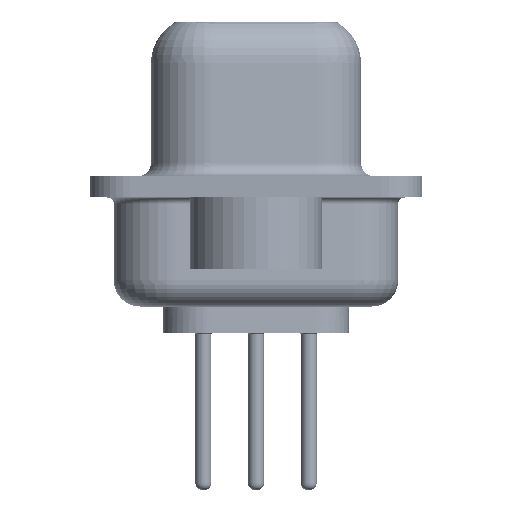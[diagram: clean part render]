
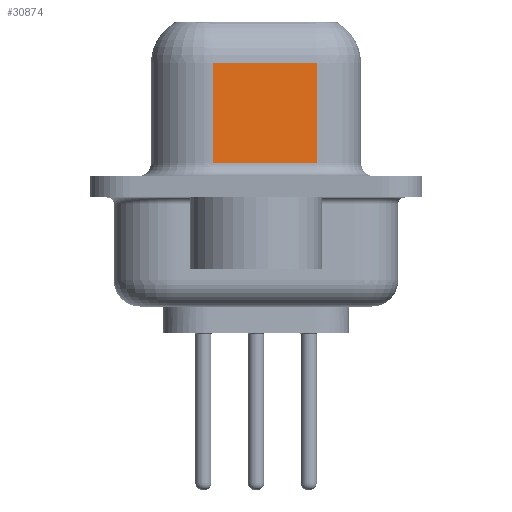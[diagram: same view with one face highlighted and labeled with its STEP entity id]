
A CAD part, left-side view. The second image highlights one B-rep face of the part: STEP entity #30874.
In plain terms, the highlighted planar face has unit normal (-0.985, -0.174, 0).
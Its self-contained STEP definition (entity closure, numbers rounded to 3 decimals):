
#3888 = EDGE_CURVE ( 'NONE', #25806, #20853, #15458, .T. ) ;
#4741 = ORIENTED_EDGE ( 'NONE', *, *, #3888, .T. ) ;
#5418 = FACE_OUTER_BOUND ( 'NONE', #9140, .T. ) ;
#7743 = AXIS2_PLACEMENT_3D ( 'NONE', #19581, #20335, #17105 ) ;
#7996 = CARTESIAN_POINT ( 'NONE',  ( 5.068, -2.297, 4.65 ) ) ;
#8545 = EDGE_CURVE ( 'NONE', #13264, #25353, #14370, .T. ) ;
#8855 = LINE ( 'NONE', #32170, #36626 ) ;
#9140 = EDGE_LOOP ( 'NONE', ( #12347, #4741, #17244, #30622 ) ) ;
#9578 = VECTOR ( 'NONE', #24251, 1000. ) ;
#12347 = ORIENTED_EDGE ( 'NONE', *, *, #23594, .F. ) ;
#13264 = VERTEX_POINT ( 'NONE', #17322 ) ;
#14370 = LINE ( 'NONE', #16671, #29075 ) ;
#14899 = CARTESIAN_POINT ( 'NONE',  ( 5.068, -2.297, 4.65 ) ) ;
#15458 = LINE ( 'NONE', #14899, #9578 ) ;
#15962 = CARTESIAN_POINT ( 'NONE',  ( 5.068, -2.297, 6.4 ) ) ;
#16671 = CARTESIAN_POINT ( 'NONE',  ( 5.068, -2.297, 0.9 ) ) ;
#16853 = CARTESIAN_POINT ( 'NONE',  ( 5.068, -2.297, 0.9 ) ) ;
#17105 = DIRECTION ( 'NONE',  ( -0.174, 0.985, 0. ) ) ;
#17244 = ORIENTED_EDGE ( 'NONE', *, *, #20982, .T. ) ;
#17322 = CARTESIAN_POINT ( 'NONE',  ( 4.38, 1.603, 0.9 ) ) ;
#19581 = CARTESIAN_POINT ( 'NONE',  ( 5.068, -2.297, 6.4 ) ) ;
#20335 = DIRECTION ( 'NONE',  ( 0.985, 0.174, 0. ) ) ;
#20853 = VERTEX_POINT ( 'NONE', #37315 ) ;
#20982 = EDGE_CURVE ( 'NONE', #20853, #13264, #8855, .T. ) ;
#22970 = DIRECTION ( 'NONE',  ( 0.174, -0.985, 0. ) ) ;
#23594 = EDGE_CURVE ( 'NONE', #25806, #25353, #27783, .T. ) ;
#24251 = DIRECTION ( 'NONE',  ( -0.174, 0.985, 0. ) ) ;
#24920 = DIRECTION ( 'NONE',  ( 0., 0., -1. ) ) ;
#25353 = VERTEX_POINT ( 'NONE', #16853 ) ;
#25806 = VERTEX_POINT ( 'NONE', #7996 ) ;
#27783 = LINE ( 'NONE', #15962, #29410 ) ;
#28538 = PLANE ( 'NONE',  #7743 ) ;
#29075 = VECTOR ( 'NONE', #22970, 1000. ) ;
#29410 = VECTOR ( 'NONE', #24920, 1000. ) ;
#29874 = DIRECTION ( 'NONE',  ( 0., 0., -1. ) ) ;
#30622 = ORIENTED_EDGE ( 'NONE', *, *, #8545, .T. ) ;
#30874 = ADVANCED_FACE ( 'NONE', ( #5418 ), #28538, .F. ) ;
#32170 = CARTESIAN_POINT ( 'NONE',  ( 4.38, 1.603, 6.4 ) ) ;
#36626 = VECTOR ( 'NONE', #29874, 1000. ) ;
#37315 = CARTESIAN_POINT ( 'NONE',  ( 4.38, 1.603, 4.65 ) ) ;
